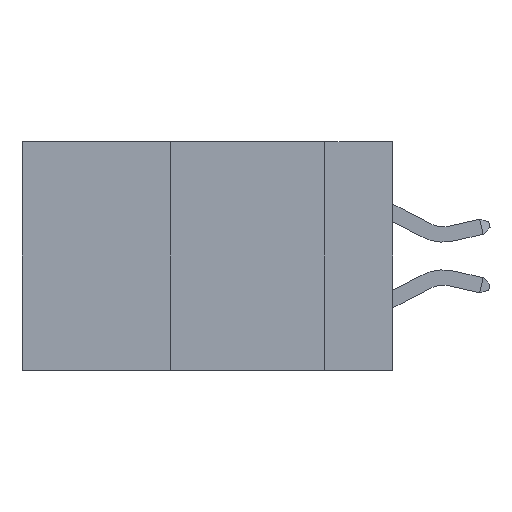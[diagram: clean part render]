
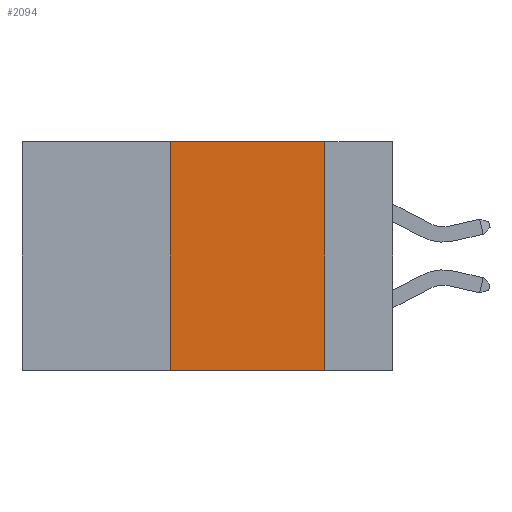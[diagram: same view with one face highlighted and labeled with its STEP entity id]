
A CAD part, left-side view. The second image highlights one B-rep face of the part: STEP entity #2094.
In plain terms, the highlighted planar face has unit normal (-1, 0, 0).
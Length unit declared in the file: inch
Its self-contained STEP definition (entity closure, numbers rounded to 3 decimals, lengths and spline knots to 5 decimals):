
#222 = AXIS2_PLACEMENT_3D ( 'NONE', #9539, #3959, #9252 ) ;
#320 = VERTEX_POINT ( 'NONE', #430 ) ;
#430 = CARTESIAN_POINT ( 'NONE',  ( 0., 0.11, -0.37 ) ) ;
#1009 = DIRECTION ( 'NONE',  ( 0., -1., 0. ) ) ;
#1993 = CARTESIAN_POINT ( 'NONE',  ( 0., 0.36, 0. ) ) ;
#2094 = ADVANCED_FACE ( 'NONE', ( #2611 ), #13439, .F. ) ;
#2184 = ORIENTED_EDGE ( 'NONE', *, *, #7911, .F. ) ;
#2566 = ORIENTED_EDGE ( 'NONE', *, *, #8419, .T. ) ;
#2582 = CARTESIAN_POINT ( 'NONE',  ( 0., 0.11, 0. ) ) ;
#2611 = FACE_OUTER_BOUND ( 'NONE', #3810, .T. ) ;
#3172 = DIRECTION ( 'NONE',  ( 0., 0., 1. ) ) ;
#3530 = LINE ( 'NONE', #9909, #6125 ) ;
#3810 = EDGE_LOOP ( 'NONE', ( #2184, #5221, #8166, #2566 ) ) ;
#3896 = EDGE_CURVE ( 'NONE', #12549, #9707, #13170, .T. ) ;
#3959 = DIRECTION ( 'NONE',  ( 1., 0., 0. ) ) ;
#4602 = LINE ( 'NONE', #1993, #7149 ) ;
#4889 = VECTOR ( 'NONE', #5034, 39.37008 ) ;
#5034 = DIRECTION ( 'NONE',  ( 0., -1., 0. ) ) ;
#5221 = ORIENTED_EDGE ( 'NONE', *, *, #3896, .F. ) ;
#5468 = VECTOR ( 'NONE', #9219, 39.37008 ) ;
#5793 = CARTESIAN_POINT ( 'NONE',  ( 0., 0.6, 0. ) ) ;
#5856 = CARTESIAN_POINT ( 'NONE',  ( 0., 0.36, -0.37 ) ) ;
#6125 = VECTOR ( 'NONE', #1009, 39.37008 ) ;
#6163 = VERTEX_POINT ( 'NONE', #5856 ) ;
#7149 = VECTOR ( 'NONE', #3172, 39.37008 ) ;
#7911 = EDGE_CURVE ( 'NONE', #9707, #320, #13622, .T. ) ;
#8095 = CARTESIAN_POINT ( 'NONE',  ( 0., 0.11, 0. ) ) ;
#8166 = ORIENTED_EDGE ( 'NONE', *, *, #8276, .F. ) ;
#8276 = EDGE_CURVE ( 'NONE', #6163, #12549, #4602, .T. ) ;
#8419 = EDGE_CURVE ( 'NONE', #6163, #320, #3530, .T. ) ;
#9219 = DIRECTION ( 'NONE',  ( 0., 0., -1. ) ) ;
#9252 = DIRECTION ( 'NONE',  ( 0., 0., -1. ) ) ;
#9539 = CARTESIAN_POINT ( 'NONE',  ( 0., 0.6, 0. ) ) ;
#9707 = VERTEX_POINT ( 'NONE', #2582 ) ;
#9909 = CARTESIAN_POINT ( 'NONE',  ( 0., 0.6, -0.37 ) ) ;
#11401 = CARTESIAN_POINT ( 'NONE',  ( 0., 0.36, 0. ) ) ;
#12549 = VERTEX_POINT ( 'NONE', #11401 ) ;
#13170 = LINE ( 'NONE', #5793, #4889 ) ;
#13439 = PLANE ( 'NONE',  #222 ) ;
#13622 = LINE ( 'NONE', #8095, #5468 ) ;
